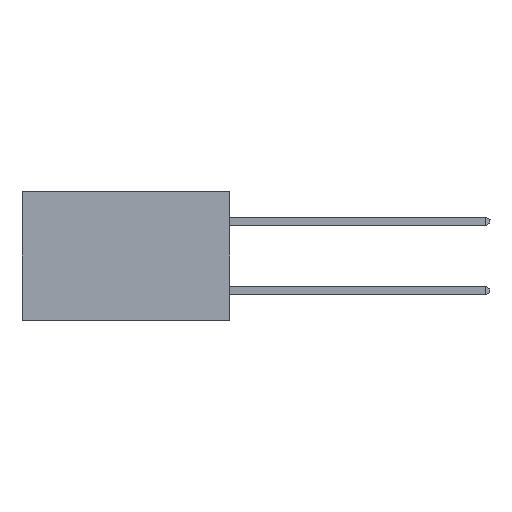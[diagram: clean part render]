
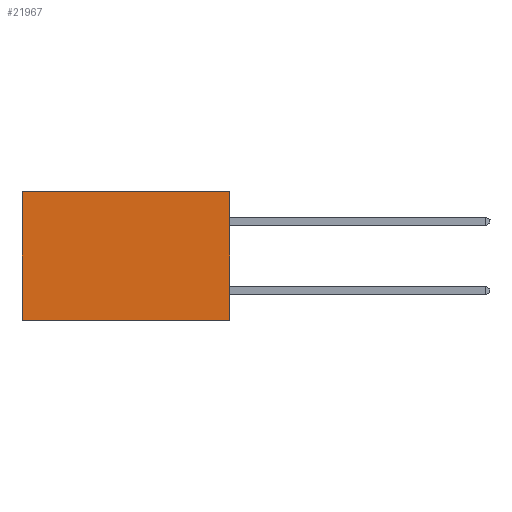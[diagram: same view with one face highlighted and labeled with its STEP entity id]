
A CAD part, left-side view. The second image highlights one B-rep face of the part: STEP entity #21967.
In plain terms, the highlighted planar face has unit normal (-1, 0, 0).
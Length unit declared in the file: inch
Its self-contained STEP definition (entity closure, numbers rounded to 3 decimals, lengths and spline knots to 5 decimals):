
#156 = CARTESIAN_POINT ( 'NONE',  ( 0.298, 0.6, 0. ) ) ;
#292 = PLANE ( 'NONE',  #10675 ) ;
#346 = FACE_OUTER_BOUND ( 'NONE', #3608, .T. ) ;
#1321 = VECTOR ( 'NONE', #24025, 39.37008 ) ;
#2128 = CARTESIAN_POINT ( 'NONE',  ( 0.298, 0., 0. ) ) ;
#3268 = DIRECTION ( 'NONE',  ( 0., 1., 0. ) ) ;
#3334 = CARTESIAN_POINT ( 'NONE',  ( 0.298, 0., -0.37 ) ) ;
#3608 = EDGE_LOOP ( 'NONE', ( #5772, #13944, #9509, #13710 ) ) ;
#3745 = VERTEX_POINT ( 'NONE', #12166 ) ;
#4082 = LINE ( 'NONE', #18102, #8867 ) ;
#4211 = EDGE_CURVE ( 'NONE', #3745, #13740, #7992, .T. ) ;
#4985 = EDGE_CURVE ( 'NONE', #16097, #3745, #14134, .T. ) ;
#5772 = ORIENTED_EDGE ( 'NONE', *, *, #23648, .T. ) ;
#7992 = LINE ( 'NONE', #3334, #1321 ) ;
#8679 = VECTOR ( 'NONE', #12433, 39.37008 ) ;
#8867 = VECTOR ( 'NONE', #20424, 39.37008 ) ;
#9370 = CARTESIAN_POINT ( 'NONE',  ( 0.298, 0., 0. ) ) ;
#9509 = ORIENTED_EDGE ( 'NONE', *, *, #4985, .F. ) ;
#10127 = DIRECTION ( 'NONE',  ( 0., 0., -1. ) ) ;
#10675 = AXIS2_PLACEMENT_3D ( 'NONE', #22661, #14443, #10127 ) ;
#10846 = CARTESIAN_POINT ( 'NONE',  ( 0.298, 0.6, -0.37 ) ) ;
#10979 = VECTOR ( 'NONE', #3268, 39.37008 ) ;
#11041 = EDGE_CURVE ( 'NONE', #16097, #20190, #17087, .T. ) ;
#12166 = CARTESIAN_POINT ( 'NONE',  ( 0.298, 0., -0.37 ) ) ;
#12433 = DIRECTION ( 'NONE',  ( 0., 0., -1. ) ) ;
#13710 = ORIENTED_EDGE ( 'NONE', *, *, #11041, .T. ) ;
#13740 = VERTEX_POINT ( 'NONE', #10846 ) ;
#13944 = ORIENTED_EDGE ( 'NONE', *, *, #4211, .F. ) ;
#14134 = LINE ( 'NONE', #2128, #8679 ) ;
#14443 = DIRECTION ( 'NONE',  ( 1., 0., 0. ) ) ;
#16097 = VERTEX_POINT ( 'NONE', #9370 ) ;
#17087 = LINE ( 'NONE', #26036, #10979 ) ;
#18102 = CARTESIAN_POINT ( 'NONE',  ( 0.298, 0.6, 0. ) ) ;
#20190 = VERTEX_POINT ( 'NONE', #156 ) ;
#20424 = DIRECTION ( 'NONE',  ( 0., 0., -1. ) ) ;
#21967 = ADVANCED_FACE ( 'NONE', ( #346 ), #292, .F. ) ;
#22661 = CARTESIAN_POINT ( 'NONE',  ( 0.298, 0., 0. ) ) ;
#23648 = EDGE_CURVE ( 'NONE', #20190, #13740, #4082, .T. ) ;
#24025 = DIRECTION ( 'NONE',  ( 0., 1., 0. ) ) ;
#26036 = CARTESIAN_POINT ( 'NONE',  ( 0.298, 0., 0. ) ) ;
